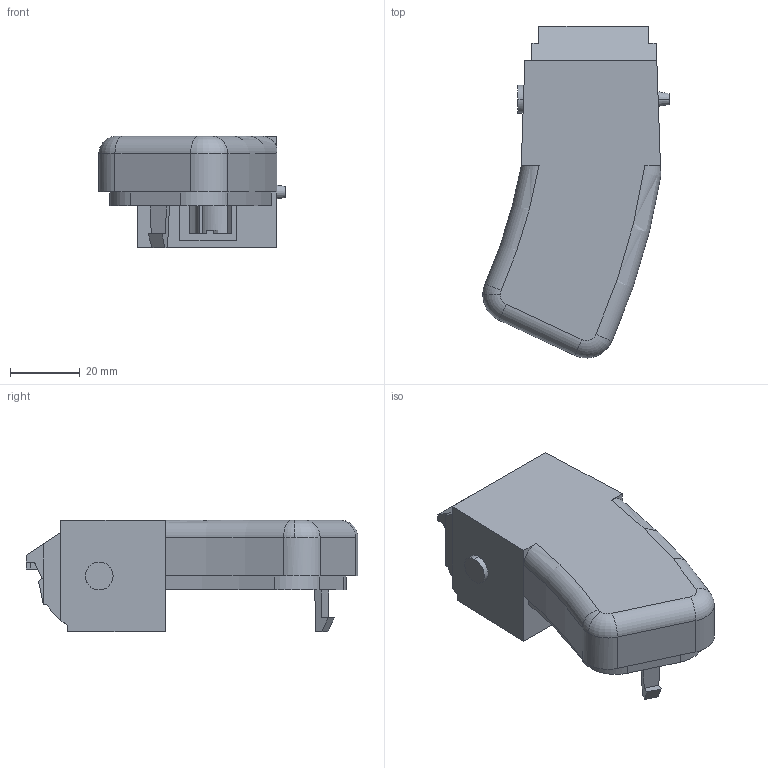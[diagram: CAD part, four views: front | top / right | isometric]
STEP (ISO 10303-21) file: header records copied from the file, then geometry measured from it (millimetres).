
FILE_DESCRIPTION (( 'STEP AP214' ), '1' );
FILE_NAME ('right_small.STEP', '2013-07-01T00:26:31', ( '' ), ( '' ), 'SwSTEP 2.0', 'SolidWorks 2013', '' );
FILE_SCHEMA (( 'AUTOMOTIVE_DESIGN' ));
Length unit declared in the file: millimetre
Products named in the file (1): right_small
Bounding box: 53.52 x 95.38 x 32 mm (x, y, z)
Volume: 51159 mm3; surface area: 22079.2 mm2
Topology: 1 solids, 1 shells, 160 faces, 451 edges, 294 vertices
Faces by surface type: plane 97, cylinder 48, torus 10, bspline 3, cone 2
Entity records: 5361 total; most frequent: CARTESIAN_POINT 1175, ORIENTED_EDGE 902, DIRECTION 852, EDGE_CURVE 451, VECTOR 296, LINE 296, VERTEX_POINT 294, AXIS2_PLACEMENT_3D 278
